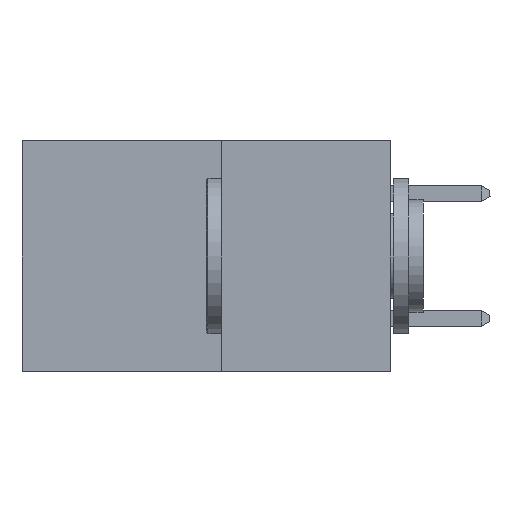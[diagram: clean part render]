
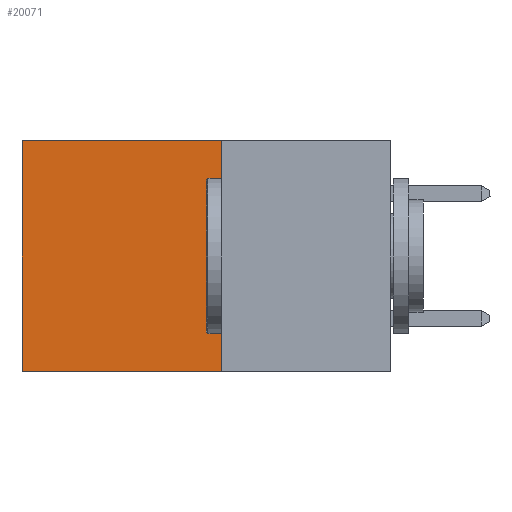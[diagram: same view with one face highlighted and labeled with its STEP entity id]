
A CAD part, left-side view. The second image highlights one B-rep face of the part: STEP entity #20071.
In plain terms, the highlighted planar face has unit normal (-1, 0, 0).
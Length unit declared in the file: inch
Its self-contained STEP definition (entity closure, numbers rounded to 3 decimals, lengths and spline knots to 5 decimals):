
#175 = CARTESIAN_POINT ( 'NONE',  ( 0.277, 0.27, -0.37 ) ) ;
#295 = VECTOR ( 'NONE', #11382, 39.37008 ) ;
#655 = VERTEX_POINT ( 'NONE', #13513 ) ;
#1401 = VECTOR ( 'NONE', #4950, 39.37008 ) ;
#1876 = ORIENTED_EDGE ( 'NONE', *, *, #23653, .F. ) ;
#2064 = LINE ( 'NONE', #17234, #1401 ) ;
#2355 = ORIENTED_EDGE ( 'NONE', *, *, #11631, .F. ) ;
#3784 = CARTESIAN_POINT ( 'NONE',  ( 0.277, 0.59, 0. ) ) ;
#4821 = EDGE_LOOP ( 'NONE', ( #24616, #1876, #2355, #5574 ) ) ;
#4906 = LINE ( 'NONE', #13726, #25964 ) ;
#4950 = DIRECTION ( 'NONE',  ( 0., 1., 0. ) ) ;
#5574 = ORIENTED_EDGE ( 'NONE', *, *, #12002, .T. ) ;
#5880 = LINE ( 'NONE', #7226, #295 ) ;
#6134 = PLANE ( 'NONE',  #25452 ) ;
#7226 = CARTESIAN_POINT ( 'NONE',  ( 0.277, 0.59, -0.37 ) ) ;
#8224 = DIRECTION ( 'NONE',  ( 1., 0., 0. ) ) ;
#9258 = VERTEX_POINT ( 'NONE', #3784 ) ;
#11382 = DIRECTION ( 'NONE',  ( 0., 0., -1. ) ) ;
#11631 = EDGE_CURVE ( 'NONE', #13425, #16162, #18753, .T. ) ;
#12002 = EDGE_CURVE ( 'NONE', #13425, #9258, #4906, .T. ) ;
#13425 = VERTEX_POINT ( 'NONE', #20737 ) ;
#13513 = CARTESIAN_POINT ( 'NONE',  ( 0.277, 0.59, -0.37 ) ) ;
#13726 = CARTESIAN_POINT ( 'NONE',  ( 0.277, 0.27, 0. ) ) ;
#14381 = CARTESIAN_POINT ( 'NONE',  ( 0.277, 0.27, -0.37 ) ) ;
#16162 = VERTEX_POINT ( 'NONE', #20795 ) ;
#17234 = CARTESIAN_POINT ( 'NONE',  ( 0.277, 0.27, -0.37 ) ) ;
#18753 = LINE ( 'NONE', #175, #24093 ) ;
#19060 = FACE_OUTER_BOUND ( 'NONE', #4821, .T. ) ;
#20071 = ADVANCED_FACE ( 'NONE', ( #19060 ), #6134, .F. ) ;
#20737 = CARTESIAN_POINT ( 'NONE',  ( 0.277, 0.27, 0. ) ) ;
#20795 = CARTESIAN_POINT ( 'NONE',  ( 0.277, 0.27, -0.37 ) ) ;
#22508 = DIRECTION ( 'NONE',  ( 0., 0., -1. ) ) ;
#22778 = DIRECTION ( 'NONE',  ( 0., 0., -1. ) ) ;
#23653 = EDGE_CURVE ( 'NONE', #16162, #655, #2064, .T. ) ;
#23827 = DIRECTION ( 'NONE',  ( 0., 1., 0. ) ) ;
#24093 = VECTOR ( 'NONE', #22778, 39.37008 ) ;
#24616 = ORIENTED_EDGE ( 'NONE', *, *, #25706, .T. ) ;
#25452 = AXIS2_PLACEMENT_3D ( 'NONE', #14381, #8224, #22508 ) ;
#25706 = EDGE_CURVE ( 'NONE', #9258, #655, #5880, .T. ) ;
#25964 = VECTOR ( 'NONE', #23827, 39.37008 ) ;
